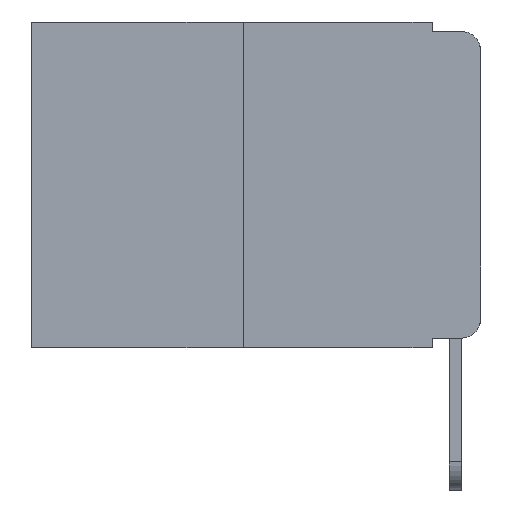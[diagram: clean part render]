
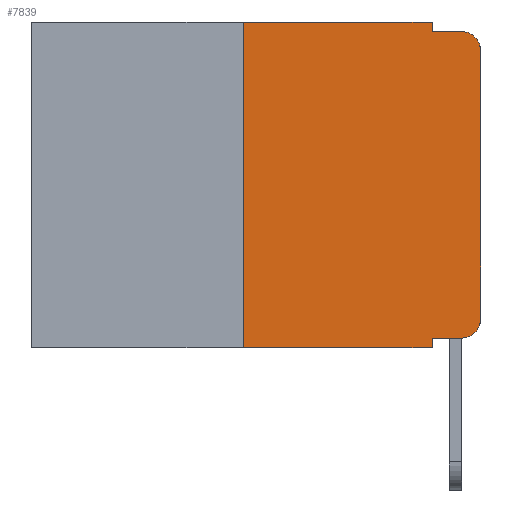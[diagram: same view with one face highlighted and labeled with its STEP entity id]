
A CAD part, left-side view. The second image highlights one B-rep face of the part: STEP entity #7839.
In plain terms, the highlighted planar face has unit normal (-1, 0, 0).
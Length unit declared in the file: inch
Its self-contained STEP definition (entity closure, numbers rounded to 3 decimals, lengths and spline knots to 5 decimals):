
#113 = PLANE ( 'NONE',  #4644 ) ;
#223 = CARTESIAN_POINT ( 'NONE',  ( 0., 0.25, 0. ) ) ;
#289 = EDGE_CURVE ( 'NONE', #10269, #3464, #1966, .T. ) ;
#395 = ORIENTED_EDGE ( 'NONE', *, *, #9743, .T. ) ;
#463 = ORIENTED_EDGE ( 'NONE', *, *, #4567, .T. ) ;
#535 = ORIENTED_EDGE ( 'NONE', *, *, #1003, .T. ) ;
#606 = VERTEX_POINT ( 'NONE', #10183 ) ;
#746 = CARTESIAN_POINT ( 'NONE',  ( 0., 0.02, -0.333 ) ) ;
#860 = ORIENTED_EDGE ( 'NONE', *, *, #4762, .T. ) ;
#965 = CARTESIAN_POINT ( 'NONE',  ( 0., 0.25, 0. ) ) ;
#1003 = EDGE_CURVE ( 'NONE', #3770, #606, #4279, .T. ) ;
#1104 = CARTESIAN_POINT ( 'NONE',  ( 0., 0.473, 0. ) ) ;
#1129 = CARTESIAN_POINT ( 'NONE',  ( 0., 0.25, -0.343 ) ) ;
#1563 = ORIENTED_EDGE ( 'NONE', *, *, #289, .F. ) ;
#1602 = CARTESIAN_POINT ( 'NONE',  ( 0., 0.051, -0.333 ) ) ;
#1795 = DIRECTION ( 'NONE',  ( 0., -1., 0. ) ) ;
#1966 = LINE ( 'NONE', #4744, #9105 ) ;
#2290 = EDGE_CURVE ( 'NONE', #11711, #9018, #9467, .T. ) ;
#2341 = CIRCLE ( 'NONE', #9814, 0.02 ) ;
#2559 = LINE ( 'NONE', #1602, #3250 ) ;
#2866 = LINE ( 'NONE', #965, #10178 ) ;
#2910 = DIRECTION ( 'NONE',  ( 0., -1., 0. ) ) ;
#2944 = EDGE_CURVE ( 'NONE', #3404, #4265, #2866, .T. ) ;
#3050 = DIRECTION ( 'NONE',  ( 0., 0., 1. ) ) ;
#3250 = VECTOR ( 'NONE', #1795, 39.37008 ) ;
#3404 = VERTEX_POINT ( 'NONE', #1129 ) ;
#3464 = VERTEX_POINT ( 'NONE', #5824 ) ;
#3594 = CARTESIAN_POINT ( 'NONE',  ( 0., 0., -0.313 ) ) ;
#3600 = CARTESIAN_POINT ( 'NONE',  ( 0., 0.473, 0. ) ) ;
#3722 = LINE ( 'NONE', #11433, #10427 ) ;
#3770 = VERTEX_POINT ( 'NONE', #3594 ) ;
#3865 = LINE ( 'NONE', #7738, #8840 ) ;
#4265 = VERTEX_POINT ( 'NONE', #223 ) ;
#4279 = LINE ( 'NONE', #6308, #6199 ) ;
#4567 = EDGE_CURVE ( 'NONE', #606, #9735, #10858, .T. ) ;
#4644 = AXIS2_PLACEMENT_3D ( 'NONE', #1104, #6936, #7944 ) ;
#4744 = CARTESIAN_POINT ( 'NONE',  ( 0., 0.051, 0. ) ) ;
#4762 = EDGE_CURVE ( 'NONE', #3404, #9018, #3865, .T. ) ;
#5431 = VERTEX_POINT ( 'NONE', #746 ) ;
#5506 = DIRECTION ( 'NONE',  ( 0., -1., 0. ) ) ;
#5560 = LINE ( 'NONE', #3600, #6640 ) ;
#5820 = DIRECTION ( 'NONE',  ( 0., 0., -1. ) ) ;
#5824 = CARTESIAN_POINT ( 'NONE',  ( 0., 0.051, -0.01 ) ) ;
#6159 = ORIENTED_EDGE ( 'NONE', *, *, #6716, .F. ) ;
#6199 = VECTOR ( 'NONE', #7140, 39.37008 ) ;
#6252 = DIRECTION ( 'NONE',  ( -1., 0., 0. ) ) ;
#6308 = CARTESIAN_POINT ( 'NONE',  ( 0., 0., 0. ) ) ;
#6417 = CARTESIAN_POINT ( 'NONE',  ( 0., 0.02, -0.01 ) ) ;
#6566 = DIRECTION ( 'NONE',  ( 0., 0., -1. ) ) ;
#6570 = ORIENTED_EDGE ( 'NONE', *, *, #2290, .F. ) ;
#6637 = DIRECTION ( 'NONE',  ( 0., -1., 0. ) ) ;
#6640 = VECTOR ( 'NONE', #5506, 39.37008 ) ;
#6716 = EDGE_CURVE ( 'NONE', #4265, #10269, #5560, .T. ) ;
#6936 = DIRECTION ( 'NONE',  ( 1., 0., 0. ) ) ;
#7140 = DIRECTION ( 'NONE',  ( 0., 0., 1. ) ) ;
#7213 = DIRECTION ( 'NONE',  ( 0., 0., -1. ) ) ;
#7469 = CARTESIAN_POINT ( 'NONE',  ( 0., 0.051, 0. ) ) ;
#7738 = CARTESIAN_POINT ( 'NONE',  ( 0., 0.473, -0.343 ) ) ;
#7839 = ADVANCED_FACE ( 'NONE', ( #8767 ), #113, .F. ) ;
#7944 = DIRECTION ( 'NONE',  ( 0., 0., -1. ) ) ;
#8659 = CARTESIAN_POINT ( 'NONE',  ( 0., 0.051, -0.333 ) ) ;
#8700 = ORIENTED_EDGE ( 'NONE', *, *, #2944, .F. ) ;
#8767 = FACE_OUTER_BOUND ( 'NONE', #11318, .T. ) ;
#8770 = CARTESIAN_POINT ( 'NONE',  ( 0., 0.051, 0. ) ) ;
#8840 = VECTOR ( 'NONE', #2910, 39.37008 ) ;
#9018 = VERTEX_POINT ( 'NONE', #11608 ) ;
#9074 = VECTOR ( 'NONE', #6566, 39.37008 ) ;
#9105 = VECTOR ( 'NONE', #5820, 39.37008 ) ;
#9372 = DIRECTION ( 'NONE',  ( -1., 0., 0. ) ) ;
#9467 = LINE ( 'NONE', #7469, #9074 ) ;
#9735 = VERTEX_POINT ( 'NONE', #6417 ) ;
#9743 = EDGE_CURVE ( 'NONE', #11711, #5431, #2559, .T. ) ;
#9814 = AXIS2_PLACEMENT_3D ( 'NONE', #11189, #6252, #7213 ) ;
#10178 = VECTOR ( 'NONE', #3050, 39.37008 ) ;
#10183 = CARTESIAN_POINT ( 'NONE',  ( 0., 0., -0.03 ) ) ;
#10269 = VERTEX_POINT ( 'NONE', #8770 ) ;
#10427 = VECTOR ( 'NONE', #6637, 39.37008 ) ;
#10515 = DIRECTION ( 'NONE',  ( 0., 0., -1. ) ) ;
#10526 = ORIENTED_EDGE ( 'NONE', *, *, #11505, .T. ) ;
#10858 = CIRCLE ( 'NONE', #11272, 0.02 ) ;
#11189 = CARTESIAN_POINT ( 'NONE',  ( 0., 0.02, -0.313 ) ) ;
#11272 = AXIS2_PLACEMENT_3D ( 'NONE', #11396, #9372, #10515 ) ;
#11318 = EDGE_LOOP ( 'NONE', ( #535, #463, #11445, #1563, #6159, #8700, #860, #6570, #395, #10526 ) ) ;
#11396 = CARTESIAN_POINT ( 'NONE',  ( 0., 0.02, -0.03 ) ) ;
#11433 = CARTESIAN_POINT ( 'NONE',  ( 0., 0.051, -0.01 ) ) ;
#11445 = ORIENTED_EDGE ( 'NONE', *, *, #11730, .F. ) ;
#11505 = EDGE_CURVE ( 'NONE', #5431, #3770, #2341, .T. ) ;
#11608 = CARTESIAN_POINT ( 'NONE',  ( 0., 0.051, -0.343 ) ) ;
#11711 = VERTEX_POINT ( 'NONE', #8659 ) ;
#11730 = EDGE_CURVE ( 'NONE', #3464, #9735, #3722, .T. ) ;
